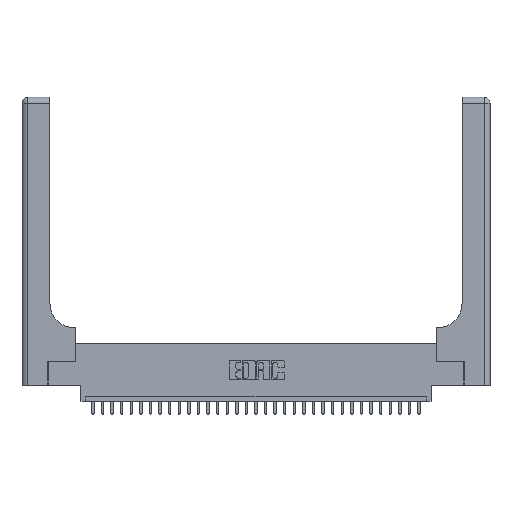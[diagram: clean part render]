
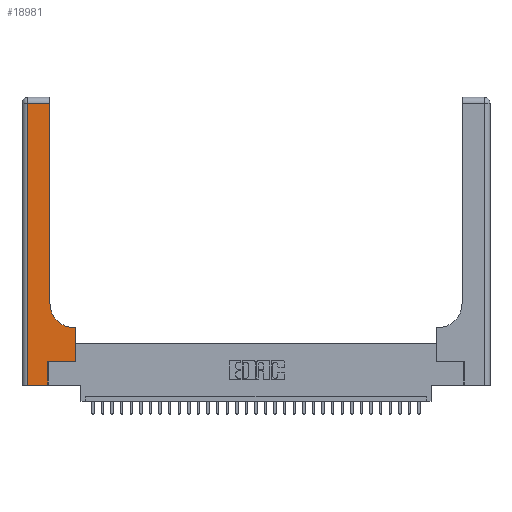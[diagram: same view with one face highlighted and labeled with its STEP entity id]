
A CAD part, top view. The second image highlights one B-rep face of the part: STEP entity #18981.
In plain terms, the highlighted planar face has unit normal (0, 0, 1).
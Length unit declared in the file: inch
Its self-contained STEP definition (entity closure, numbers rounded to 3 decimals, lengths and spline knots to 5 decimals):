
#799 = LINE ( 'NONE', #13482, #12173 ) ;
#1611 = DIRECTION ( 'NONE',  ( 1., 0., 0. ) ) ;
#1835 = CIRCLE ( 'NONE', #6708, 0.25 ) ;
#2550 = EDGE_CURVE ( 'NONE', #3418, #26407, #10261, .T. ) ;
#2576 = VECTOR ( 'NONE', #26517, 39.37008 ) ;
#2596 = CARTESIAN_POINT ( 'NONE',  ( 0.5415, 0.85, 0.37 ) ) ;
#3053 = VECTOR ( 'NONE', #17076, 39.37008 ) ;
#3418 = VERTEX_POINT ( 'NONE', #12084 ) ;
#3988 = CARTESIAN_POINT ( 'NONE',  ( 0.06, 0., 0.37 ) ) ;
#5649 = DIRECTION ( 'NONE',  ( 0., -1., 0. ) ) ;
#5841 = EDGE_CURVE ( 'NONE', #25976, #3418, #16010, .T. ) ;
#6224 = CARTESIAN_POINT ( 'NONE',  ( 0., 2.94, 0.37 ) ) ;
#6708 = AXIS2_PLACEMENT_3D ( 'NONE', #2596, #20243, #7659 ) ;
#7659 = DIRECTION ( 'NONE',  ( 1., 0., 0. ) ) ;
#7897 = CARTESIAN_POINT ( 'NONE',  ( 0.06, 2.94, 0.37 ) ) ;
#8289 = EDGE_CURVE ( 'NONE', #23082, #23369, #19774, .T. ) ;
#8617 = DIRECTION ( 'NONE',  ( 0., 1., 0. ) ) ;
#9670 = LINE ( 'NONE', #6224, #2576 ) ;
#9910 = EDGE_CURVE ( 'NONE', #23369, #31842, #16967, .T. ) ;
#10261 = LINE ( 'NONE', #19955, #19790 ) ;
#11038 = EDGE_CURVE ( 'NONE', #31842, #15380, #31373, .T. ) ;
#12084 = CARTESIAN_POINT ( 'NONE',  ( 0.5585, 0.6, 0.37 ) ) ;
#12173 = VECTOR ( 'NONE', #18475, 39.37008 ) ;
#12316 = ORIENTED_EDGE ( 'NONE', *, *, #11038, .T. ) ;
#13482 = CARTESIAN_POINT ( 'NONE',  ( 0.2915, 3., 0.37 ) ) ;
#13819 = CARTESIAN_POINT ( 'NONE',  ( 0.5585, 0.25, 0.37 ) ) ;
#14772 = DIRECTION ( 'NONE',  ( 0., 1., 0. ) ) ;
#15055 = ORIENTED_EDGE ( 'NONE', *, *, #2550, .T. ) ;
#15297 = LINE ( 'NONE', #32264, #3053 ) ;
#15380 = VERTEX_POINT ( 'NONE', #23584 ) ;
#15586 = CARTESIAN_POINT ( 'NONE',  ( 0., 3., 0.37 ) ) ;
#16010 = LINE ( 'NONE', #13819, #28606 ) ;
#16033 = ORIENTED_EDGE ( 'NONE', *, *, #30803, .T. ) ;
#16043 = ORIENTED_EDGE ( 'NONE', *, *, #8289, .T. ) ;
#16826 = VECTOR ( 'NONE', #14772, 39.37008 ) ;
#16967 = LINE ( 'NONE', #26824, #31941 ) ;
#17076 = DIRECTION ( 'NONE',  ( 1., 0., 0. ) ) ;
#17546 = CARTESIAN_POINT ( 'NONE',  ( 0.269, 0., 0.37 ) ) ;
#17622 = EDGE_CURVE ( 'NONE', #15380, #25976, #15297, .T. ) ;
#18019 = DIRECTION ( 'NONE',  ( -1., 0., 0. ) ) ;
#18047 = ORIENTED_EDGE ( 'NONE', *, *, #5841, .T. ) ;
#18475 = DIRECTION ( 'NONE',  ( 0., 1., 0. ) ) ;
#18665 = EDGE_CURVE ( 'NONE', #29761, #23082, #9670, .T. ) ;
#18981 = ADVANCED_FACE ( 'NONE', ( #26236 ), #30765, .F. ) ;
#19774 = LINE ( 'NONE', #28047, #30777 ) ;
#19790 = VECTOR ( 'NONE', #20161, 39.37008 ) ;
#19955 = CARTESIAN_POINT ( 'NONE',  ( 0.2915, 0.6, 0.37 ) ) ;
#20161 = DIRECTION ( 'NONE',  ( -1., 0., 0. ) ) ;
#20243 = DIRECTION ( 'NONE',  ( 0., 0., -1. ) ) ;
#20784 = ORIENTED_EDGE ( 'NONE', *, *, #9910, .T. ) ;
#22607 = EDGE_LOOP ( 'NONE', ( #16033, #24160, #16043, #20784, #12316, #25734, #18047, #15055, #26568 ) ) ;
#23082 = VERTEX_POINT ( 'NONE', #7897 ) ;
#23369 = VERTEX_POINT ( 'NONE', #3988 ) ;
#23584 = CARTESIAN_POINT ( 'NONE',  ( 0.269, 0.25, 0.37 ) ) ;
#24078 = CARTESIAN_POINT ( 'NONE',  ( 0.2915, 2.94, 0.37 ) ) ;
#24160 = ORIENTED_EDGE ( 'NONE', *, *, #18665, .T. ) ;
#24308 = EDGE_CURVE ( 'NONE', #26407, #30208, #1835, .T. ) ;
#25734 = ORIENTED_EDGE ( 'NONE', *, *, #17622, .T. ) ;
#25976 = VERTEX_POINT ( 'NONE', #30097 ) ;
#26236 = FACE_OUTER_BOUND ( 'NONE', #22607, .T. ) ;
#26331 = CARTESIAN_POINT ( 'NONE',  ( 0.5415, 0.6, 0.37 ) ) ;
#26407 = VERTEX_POINT ( 'NONE', #26331 ) ;
#26517 = DIRECTION ( 'NONE',  ( -1., 0., 0. ) ) ;
#26568 = ORIENTED_EDGE ( 'NONE', *, *, #24308, .T. ) ;
#26824 = CARTESIAN_POINT ( 'NONE',  ( 0., 0., 0.37 ) ) ;
#28047 = CARTESIAN_POINT ( 'NONE',  ( 0.06, 3., 0.37 ) ) ;
#28558 = CARTESIAN_POINT ( 'NONE',  ( 0.2915, 0.85, 0.37 ) ) ;
#28606 = VECTOR ( 'NONE', #8617, 39.37008 ) ;
#29761 = VERTEX_POINT ( 'NONE', #24078 ) ;
#30097 = CARTESIAN_POINT ( 'NONE',  ( 0.5585, 0.25, 0.37 ) ) ;
#30208 = VERTEX_POINT ( 'NONE', #28558 ) ;
#30255 = AXIS2_PLACEMENT_3D ( 'NONE', #15586, #30442, #18019 ) ;
#30442 = DIRECTION ( 'NONE',  ( 0., 0., -1. ) ) ;
#30540 = CARTESIAN_POINT ( 'NONE',  ( 0.269, 0., 0.37 ) ) ;
#30765 = PLANE ( 'NONE',  #30255 ) ;
#30777 = VECTOR ( 'NONE', #5649, 39.37008 ) ;
#30803 = EDGE_CURVE ( 'NONE', #30208, #29761, #799, .T. ) ;
#31373 = LINE ( 'NONE', #30540, #16826 ) ;
#31842 = VERTEX_POINT ( 'NONE', #17546 ) ;
#31941 = VECTOR ( 'NONE', #1611, 39.37008 ) ;
#32264 = CARTESIAN_POINT ( 'NONE',  ( 0.269, 0.25, 0.37 ) ) ;
